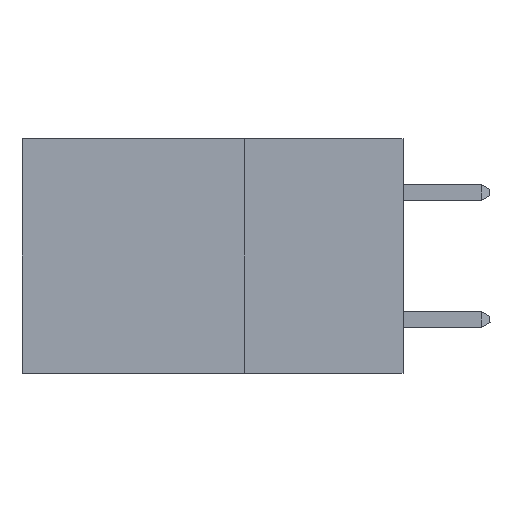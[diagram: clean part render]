
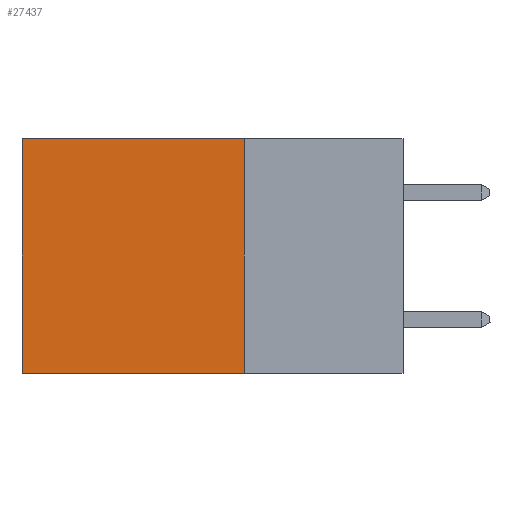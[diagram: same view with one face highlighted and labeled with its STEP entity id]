
A CAD part, left-side view. The second image highlights one B-rep face of the part: STEP entity #27437.
In plain terms, the highlighted planar face has unit normal (-1, 0, 0).
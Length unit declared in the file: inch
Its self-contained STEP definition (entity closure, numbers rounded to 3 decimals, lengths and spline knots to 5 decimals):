
#383 = VECTOR ( 'NONE', #3930, 39.37008 ) ;
#891 = LINE ( 'NONE', #18204, #20882 ) ;
#1415 = VERTEX_POINT ( 'NONE', #28369 ) ;
#2090 = VECTOR ( 'NONE', #17120, 39.37008 ) ;
#2977 = CARTESIAN_POINT ( 'NONE',  ( 0.2875, 0.6, 0. ) ) ;
#3930 = DIRECTION ( 'NONE',  ( 0., 1., 0. ) ) ;
#4462 = CARTESIAN_POINT ( 'NONE',  ( 0.2875, 0.25, -0.37 ) ) ;
#4467 = CARTESIAN_POINT ( 'NONE',  ( 0.2875, 0.6, -0.37 ) ) ;
#13560 = LINE ( 'NONE', #17109, #32263 ) ;
#14222 = PLANE ( 'NONE',  #18169 ) ;
#14993 = EDGE_LOOP ( 'NONE', ( #15961, #19173, #25804, #33114 ) ) ;
#15961 = ORIENTED_EDGE ( 'NONE', *, *, #22038, .T. ) ;
#17095 = DIRECTION ( 'NONE',  ( 1., 0., 0. ) ) ;
#17109 = CARTESIAN_POINT ( 'NONE',  ( 0.2875, 0.25, 0. ) ) ;
#17120 = DIRECTION ( 'NONE',  ( 0., 0., -1. ) ) ;
#17784 = VERTEX_POINT ( 'NONE', #34749 ) ;
#17955 = DIRECTION ( 'NONE',  ( 0., 0., -1. ) ) ;
#18169 = AXIS2_PLACEMENT_3D ( 'NONE', #34135, #17095, #33652 ) ;
#18204 = CARTESIAN_POINT ( 'NONE',  ( 0.2875, 0.25, 0. ) ) ;
#18510 = VERTEX_POINT ( 'NONE', #4462 ) ;
#18983 = EDGE_CURVE ( 'NONE', #18510, #36018, #26604, .T. ) ;
#19173 = ORIENTED_EDGE ( 'NONE', *, *, #18983, .F. ) ;
#20029 = FACE_OUTER_BOUND ( 'NONE', #14993, .T. ) ;
#20882 = VECTOR ( 'NONE', #17955, 39.37008 ) ;
#22038 = EDGE_CURVE ( 'NONE', #1415, #36018, #27416, .T. ) ;
#25804 = ORIENTED_EDGE ( 'NONE', *, *, #27696, .F. ) ;
#26604 = LINE ( 'NONE', #29524, #383 ) ;
#27416 = LINE ( 'NONE', #2977, #2090 ) ;
#27437 = ADVANCED_FACE ( 'NONE', ( #20029 ), #14222, .F. ) ;
#27696 = EDGE_CURVE ( 'NONE', #17784, #18510, #891, .T. ) ;
#28369 = CARTESIAN_POINT ( 'NONE',  ( 0.2875, 0.6, 0. ) ) ;
#29524 = CARTESIAN_POINT ( 'NONE',  ( 0.2875, 0.25, -0.37 ) ) ;
#30482 = EDGE_CURVE ( 'NONE', #17784, #1415, #13560, .T. ) ;
#32263 = VECTOR ( 'NONE', #36619, 39.37008 ) ;
#33114 = ORIENTED_EDGE ( 'NONE', *, *, #30482, .T. ) ;
#33652 = DIRECTION ( 'NONE',  ( 0., 0., -1. ) ) ;
#34135 = CARTESIAN_POINT ( 'NONE',  ( 0.2875, 0.25, 0. ) ) ;
#34749 = CARTESIAN_POINT ( 'NONE',  ( 0.2875, 0.25, 0. ) ) ;
#36018 = VERTEX_POINT ( 'NONE', #4467 ) ;
#36619 = DIRECTION ( 'NONE',  ( 0., 1., 0. ) ) ;
